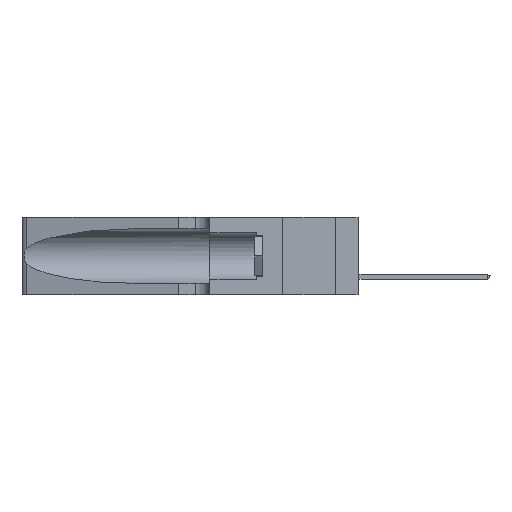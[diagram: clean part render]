
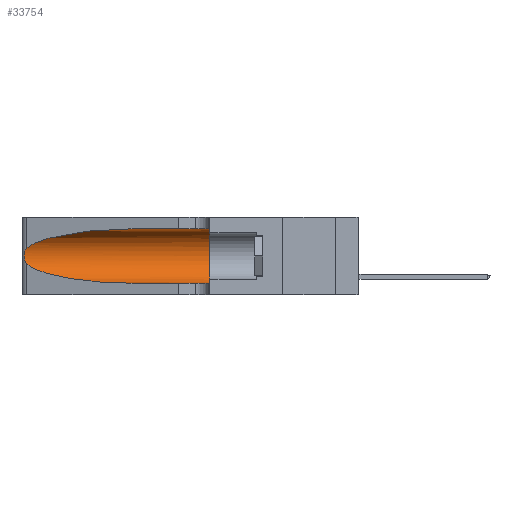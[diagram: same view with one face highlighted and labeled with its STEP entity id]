
A CAD part, left-side view. The second image highlights one B-rep face of the part: STEP entity #33754.
In plain terms, the highlighted cylindrical face has radius 3.308 mm (diameter 6.617 mm), a partial arc.
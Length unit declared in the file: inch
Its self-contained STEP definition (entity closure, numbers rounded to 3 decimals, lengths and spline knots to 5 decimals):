
#60 = EDGE_CURVE ( 'NONE', #28874, #3205, #44327, .T. ) ;
#298 = VECTOR ( 'NONE', #14625, 39.37008 ) ;
#1324 = CARTESIAN_POINT ( 'NONE',  ( 0.25487, 1.22718, 0.22369 ) ) ;
#1675 = CARTESIAN_POINT ( 'NONE',  ( 0.1305, 0.72297, 0.31525 ) ) ;
#2684 = CARTESIAN_POINT ( 'NONE',  ( 0.25854, 1.2359, 0.20912 ) ) ;
#3182 = CYLINDRICAL_SURFACE ( 'NONE', #3574, 0.13025 ) ;
#3205 = VERTEX_POINT ( 'NONE', #33991 ) ;
#3216 = ORIENTED_EDGE ( 'NONE', *, *, #60, .T. ) ;
#3259 = CARTESIAN_POINT ( 'NONE',  ( 0.25789, 1.23486, 0.15765 ) ) ;
#3574 = AXIS2_PLACEMENT_3D ( 'NONE', #9567, #24652, #5554 ) ;
#4114 = B_SPLINE_CURVE_WITH_KNOTS ( 'NONE', 3,
 ( #48911, #25491, #40552, #6406, #2684, #48360, #9188, #36947, #20085, #31517, #3259, #27163, #24451, #32435 ),
 .UNSPECIFIED., .F., .F.,
 ( 4, 2, 2, 2, 2, 2, 4 ),
 ( 0., 0.00027, 0.00053, 0.00107, 0.0016, 0.00187, 0.00214 ),
 .UNSPECIFIED. ) ;
#5554 = DIRECTION ( 'NONE',  ( 0., 0., -1. ) ) ;
#5598 = EDGE_CURVE ( 'NONE', #40537, #45937, #5947, .T. ) ;
#5947 = CIRCLE ( 'NONE', #46911, 0.13025 ) ;
#6406 = CARTESIAN_POINT ( 'NONE',  ( 0.25787, 1.23484, 0.2124 ) ) ;
#7331 = EDGE_CURVE ( 'NONE', #20358, #40537, #10307, .T. ) ;
#8572 = EDGE_LOOP ( 'NONE', ( #43870, #47695, #3216, #11209, #36487, #11983 ) ) ;
#8981 = CARTESIAN_POINT ( 'NONE',  ( 0.25487, 1.22718, 0.14631 ) ) ;
#9188 = CARTESIAN_POINT ( 'NONE',  ( 0.26075, 1.23896, 0.19203 ) ) ;
#9431 = CARTESIAN_POINT ( 'NONE',  ( 0.2373, 1.15595, 0.28018 ) ) ;
#9567 = CARTESIAN_POINT ( 'NONE',  ( 0.1305, 1.61858, 0.185 ) ) ;
#10307 = LINE ( 'NONE', #18595, #48319 ) ;
#10770 = EDGE_CURVE ( 'NONE', #3205, #45937, #31026, .T. ) ;
#11209 = ORIENTED_EDGE ( 'NONE', *, *, #10770, .T. ) ;
#11983 = ORIENTED_EDGE ( 'NONE', *, *, #7331, .F. ) ;
#14625 = DIRECTION ( 'NONE',  ( 0., -1., 0. ) ) ;
#14752 = CARTESIAN_POINT ( 'NONE',  ( 0.1305, 0.72297, 0.31525 ) ) ;
#15140 = FACE_OUTER_BOUND ( 'NONE', #8572, .T. ) ;
#18595 = CARTESIAN_POINT ( 'NONE',  ( 0.1305, 1.61858, 0.31525 ) ) ;
#19061 = EDGE_CURVE ( 'NONE', #40279, #28874, #4114, .T. ) ;
#20085 = CARTESIAN_POINT ( 'NONE',  ( 0.26017, 1.23833, 0.17102 ) ) ;
#20358 = VERTEX_POINT ( 'NONE', #14752 ) ;
#20412 = CARTESIAN_POINT ( 'NONE',  ( 0.2373, 1.15595, 0.08982 ) ) ;
#21762 = EDGE_CURVE ( 'NONE', #20358, #40279, #43581, .T. ) ;
#24451 = CARTESIAN_POINT ( 'NONE',  ( 0.25555, 1.22993, 0.14849 ) ) ;
#24652 = DIRECTION ( 'NONE',  ( 0., -1., 0. ) ) ;
#25491 = CARTESIAN_POINT ( 'NONE',  ( 0.25555, 1.22994, 0.2215 ) ) ;
#25908 = CARTESIAN_POINT ( 'NONE',  ( 0.18966, 0.96281, 0.05475 ) ) ;
#26002 = CARTESIAN_POINT ( 'NONE',  ( 0.1305, 0.35, 0.185 ) ) ;
#26958 = CARTESIAN_POINT ( 'NONE',  ( 0.1305, 0.35, 0.05475 ) ) ;
#27163 = CARTESIAN_POINT ( 'NONE',  ( 0.25639, 1.23186, 0.15144 ) ) ;
#28874 = VERTEX_POINT ( 'NONE', #8981 ) ;
#29813 = CARTESIAN_POINT ( 'NONE',  ( 0.1305, 0.72297, 0.05475 ) ) ;
#31026 = LINE ( 'NONE', #33984, #298 ) ;
#31517 = CARTESIAN_POINT ( 'NONE',  ( 0.25856, 1.23593, 0.16098 ) ) ;
#32435 = CARTESIAN_POINT ( 'NONE',  ( 0.25487, 1.22718, 0.14631 ) ) ;
#32489 = CARTESIAN_POINT ( 'NONE',  ( 0.18966, 0.96281, 0.31525 ) ) ;
#32581 = CARTESIAN_POINT ( 'NONE',  ( 0.1305, 0.35, 0.31525 ) ) ;
#33274 = DIRECTION ( 'NONE',  ( 0., 1., 0. ) ) ;
#33754 = ADVANCED_FACE ( 'NONE', ( #15140 ), #3182, .F. ) ;
#33793 = DIRECTION ( 'NONE',  ( 0., 0., 1. ) ) ;
#33984 = CARTESIAN_POINT ( 'NONE',  ( 0.1305, 1.61858, 0.05475 ) ) ;
#33991 = CARTESIAN_POINT ( 'NONE',  ( 0.1305, 0.72297, 0.05475 ) ) ;
#35682 = CARTESIAN_POINT ( 'NONE',  ( 0.25487, 1.22718, 0.14631 ) ) ;
#36487 = ORIENTED_EDGE ( 'NONE', *, *, #5598, .F. ) ;
#36947 = CARTESIAN_POINT ( 'NONE',  ( 0.26075, 1.23896, 0.178 ) ) ;
#39942 = CARTESIAN_POINT ( 'NONE',  ( 0.25487, 1.22718, 0.22369 ) ) ;
#40279 = VERTEX_POINT ( 'NONE', #39942 ) ;
#40537 = VERTEX_POINT ( 'NONE', #32581 ) ;
#40552 = CARTESIAN_POINT ( 'NONE',  ( 0.25639, 1.23184, 0.21858 ) ) ;
#43581 =( BOUNDED_CURVE ( )  B_SPLINE_CURVE ( 3, ( #1675, #32489, #9431, #1324 ),
 .UNSPECIFIED., .F., .T. ) 
 B_SPLINE_CURVE_WITH_KNOTS ( ( 4, 4 ),
 ( 1.5708, 2.84003 ),
 .UNSPECIFIED. ) 
 CURVE ( )  GEOMETRIC_REPRESENTATION_ITEM ( )  RATIONAL_B_SPLINE_CURVE ( ( 1., 0.87, 0.87, 1. ) ) 
 REPRESENTATION_ITEM ( '' )  );
#43870 = ORIENTED_EDGE ( 'NONE', *, *, #21762, .T. ) ;
#44327 =( BOUNDED_CURVE ( )  B_SPLINE_CURVE ( 3, ( #35682, #20412, #25908, #29813 ),
 .UNSPECIFIED., .F., .T. ) 
 B_SPLINE_CURVE_WITH_KNOTS ( ( 4, 4 ),
 ( 3.44316, 4.71239 ),
 .UNSPECIFIED. ) 
 CURVE ( )  GEOMETRIC_REPRESENTATION_ITEM ( )  RATIONAL_B_SPLINE_CURVE ( ( 1., 0.87, 0.87, 1. ) ) 
 REPRESENTATION_ITEM ( '' )  );
#45937 = VERTEX_POINT ( 'NONE', #26958 ) ;
#46911 = AXIS2_PLACEMENT_3D ( 'NONE', #26002, #33274, #33793 ) ;
#47695 = ORIENTED_EDGE ( 'NONE', *, *, #19061, .T. ) ;
#48319 = VECTOR ( 'NONE', #49297, 39.37008 ) ;
#48360 = CARTESIAN_POINT ( 'NONE',  ( 0.26018, 1.23835, 0.19895 ) ) ;
#48911 = CARTESIAN_POINT ( 'NONE',  ( 0.25487, 1.22718, 0.22369 ) ) ;
#49297 = DIRECTION ( 'NONE',  ( 0., -1., 0. ) ) ;
